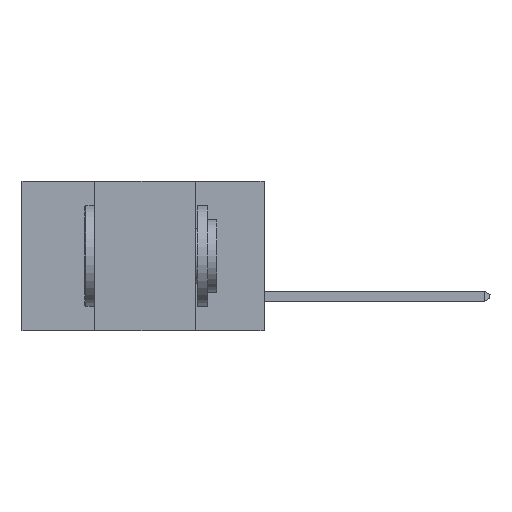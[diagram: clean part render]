
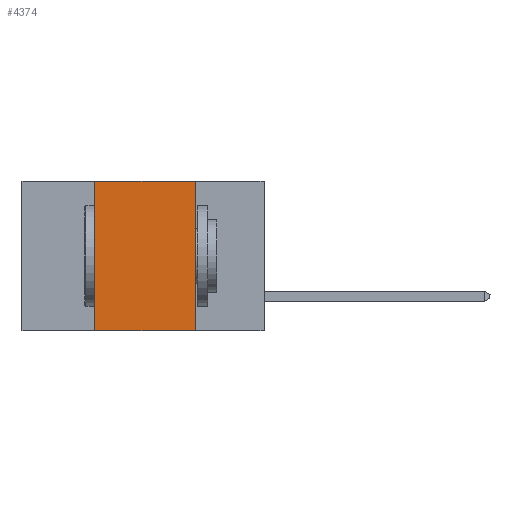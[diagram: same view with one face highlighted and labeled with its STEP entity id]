
A CAD part, left-side view. The second image highlights one B-rep face of the part: STEP entity #4374.
In plain terms, the highlighted planar face has unit normal (-1, 0, 0).
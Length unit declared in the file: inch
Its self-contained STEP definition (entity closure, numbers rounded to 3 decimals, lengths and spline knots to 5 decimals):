
#41 = LINE ( 'NONE', #2197, #7723 ) ;
#174 = DIRECTION ( 'NONE',  ( 0., 0., 1. ) ) ;
#303 = EDGE_CURVE ( 'NONE', #11269, #6277, #9381, .T. ) ;
#373 = CARTESIAN_POINT ( 'NONE',  ( 0., 0.6, -0.37 ) ) ;
#724 = DIRECTION ( 'NONE',  ( 0., 0., -1. ) ) ;
#1125 = FACE_OUTER_BOUND ( 'NONE', #2989, .T. ) ;
#2121 = VERTEX_POINT ( 'NONE', #3083 ) ;
#2197 = CARTESIAN_POINT ( 'NONE',  ( 0., 0.42, -0.37 ) ) ;
#2267 = LINE ( 'NONE', #2328, #10528 ) ;
#2288 = EDGE_CURVE ( 'NONE', #2121, #11269, #2267, .T. ) ;
#2328 = CARTESIAN_POINT ( 'NONE',  ( 0., 0.6, 0. ) ) ;
#2355 = VECTOR ( 'NONE', #724, 39.37008 ) ;
#2558 = VECTOR ( 'NONE', #4205, 39.37008 ) ;
#2633 = ORIENTED_EDGE ( 'NONE', *, *, #4698, .T. ) ;
#2672 = EDGE_CURVE ( 'NONE', #8570, #2121, #41, .T. ) ;
#2989 = EDGE_LOOP ( 'NONE', ( #5050, #5052, #11305, #2633 ) ) ;
#3083 = CARTESIAN_POINT ( 'NONE',  ( 0., 0.42, 0. ) ) ;
#4205 = DIRECTION ( 'NONE',  ( 0., -1., 0. ) ) ;
#4374 = ADVANCED_FACE ( 'NONE', ( #1125 ), #7936, .F. ) ;
#4698 = EDGE_CURVE ( 'NONE', #8570, #6277, #11118, .T. ) ;
#5050 = ORIENTED_EDGE ( 'NONE', *, *, #303, .F. ) ;
#5052 = ORIENTED_EDGE ( 'NONE', *, *, #2288, .F. ) ;
#5570 = CARTESIAN_POINT ( 'NONE',  ( 0., 0.17, -0.37 ) ) ;
#6277 = VERTEX_POINT ( 'NONE', #11457 ) ;
#6523 = AXIS2_PLACEMENT_3D ( 'NONE', #6853, #6918, #11549 ) ;
#6853 = CARTESIAN_POINT ( 'NONE',  ( 0., 0.6, 0. ) ) ;
#6918 = DIRECTION ( 'NONE',  ( 1., 0., 0. ) ) ;
#7723 = VECTOR ( 'NONE', #174, 39.37008 ) ;
#7936 = PLANE ( 'NONE',  #6523 ) ;
#8570 = VERTEX_POINT ( 'NONE', #9184 ) ;
#9184 = CARTESIAN_POINT ( 'NONE',  ( 0., 0.42, -0.37 ) ) ;
#9223 = DIRECTION ( 'NONE',  ( 0., -1., 0. ) ) ;
#9381 = LINE ( 'NONE', #5570, #2355 ) ;
#9598 = CARTESIAN_POINT ( 'NONE',  ( 0., 0.17, 0. ) ) ;
#10528 = VECTOR ( 'NONE', #9223, 39.37008 ) ;
#11118 = LINE ( 'NONE', #373, #2558 ) ;
#11269 = VERTEX_POINT ( 'NONE', #9598 ) ;
#11305 = ORIENTED_EDGE ( 'NONE', *, *, #2672, .F. ) ;
#11457 = CARTESIAN_POINT ( 'NONE',  ( 0., 0.17, -0.37 ) ) ;
#11549 = DIRECTION ( 'NONE',  ( 0., 0., -1. ) ) ;
